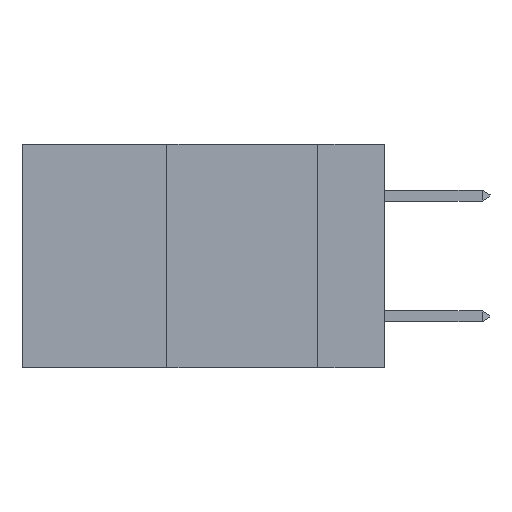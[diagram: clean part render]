
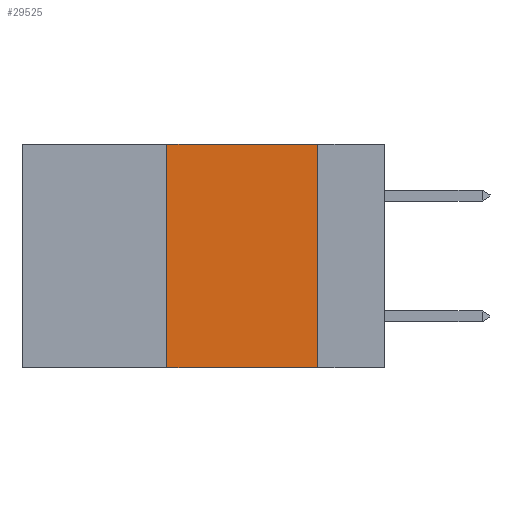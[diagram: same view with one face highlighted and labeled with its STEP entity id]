
A CAD part, left-side view. The second image highlights one B-rep face of the part: STEP entity #29525.
In plain terms, the highlighted planar face has unit normal (-1, 0, 0).
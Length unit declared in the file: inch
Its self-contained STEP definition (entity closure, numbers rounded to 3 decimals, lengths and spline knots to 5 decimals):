
#1135 = CARTESIAN_POINT ( 'NONE',  ( 0., 0.6, 0. ) ) ;
#1843 = DIRECTION ( 'NONE',  ( 0., -1., 0. ) ) ;
#1949 = VERTEX_POINT ( 'NONE', #24867 ) ;
#2465 = LINE ( 'NONE', #1135, #22121 ) ;
#3267 = EDGE_CURVE ( 'NONE', #22127, #1949, #11334, .T. ) ;
#4388 = CARTESIAN_POINT ( 'NONE',  ( 0., 0.36, -0.37 ) ) ;
#4970 = CARTESIAN_POINT ( 'NONE',  ( 0., 0.11, 0. ) ) ;
#7373 = DIRECTION ( 'NONE',  ( 1., 0., 0. ) ) ;
#7490 = ORIENTED_EDGE ( 'NONE', *, *, #21481, .F. ) ;
#7757 = EDGE_CURVE ( 'NONE', #22127, #21919, #27240, .T. ) ;
#7774 = DIRECTION ( 'NONE',  ( 0., -1., 0. ) ) ;
#7940 = LINE ( 'NONE', #4970, #17203 ) ;
#7991 = ORIENTED_EDGE ( 'NONE', *, *, #32712, .F. ) ;
#10283 = PLANE ( 'NONE',  #24839 ) ;
#11334 = LINE ( 'NONE', #22488, #17375 ) ;
#11910 = ORIENTED_EDGE ( 'NONE', *, *, #3267, .T. ) ;
#12761 = DIRECTION ( 'NONE',  ( 0., 0., 1. ) ) ;
#12909 = ORIENTED_EDGE ( 'NONE', *, *, #7757, .F. ) ;
#13035 = DIRECTION ( 'NONE',  ( 0., 0., -1. ) ) ;
#16531 = CARTESIAN_POINT ( 'NONE',  ( 0., 0.36, 0. ) ) ;
#17203 = VECTOR ( 'NONE', #13035, 39.37008 ) ;
#17375 = VECTOR ( 'NONE', #1843, 39.37008 ) ;
#17806 = CARTESIAN_POINT ( 'NONE',  ( 0., 0.6, 0. ) ) ;
#18863 = VERTEX_POINT ( 'NONE', #26565 ) ;
#20034 = VECTOR ( 'NONE', #12761, 39.37008 ) ;
#20471 = DIRECTION ( 'NONE',  ( 0., 0., -1. ) ) ;
#21481 = EDGE_CURVE ( 'NONE', #21919, #18863, #2465, .T. ) ;
#21919 = VERTEX_POINT ( 'NONE', #16531 ) ;
#22121 = VECTOR ( 'NONE', #7774, 39.37008 ) ;
#22127 = VERTEX_POINT ( 'NONE', #4388 ) ;
#22488 = CARTESIAN_POINT ( 'NONE',  ( 0., 0.6, -0.37 ) ) ;
#24732 = EDGE_LOOP ( 'NONE', ( #7991, #7490, #12909, #11910 ) ) ;
#24839 = AXIS2_PLACEMENT_3D ( 'NONE', #17806, #7373, #20471 ) ;
#24867 = CARTESIAN_POINT ( 'NONE',  ( 0., 0.11, -0.37 ) ) ;
#26565 = CARTESIAN_POINT ( 'NONE',  ( 0., 0.11, 0. ) ) ;
#27240 = LINE ( 'NONE', #27311, #20034 ) ;
#27311 = CARTESIAN_POINT ( 'NONE',  ( 0., 0.36, 0. ) ) ;
#29525 = ADVANCED_FACE ( 'NONE', ( #32216 ), #10283, .F. ) ;
#32216 = FACE_OUTER_BOUND ( 'NONE', #24732, .T. ) ;
#32712 = EDGE_CURVE ( 'NONE', #18863, #1949, #7940, .T. ) ;
